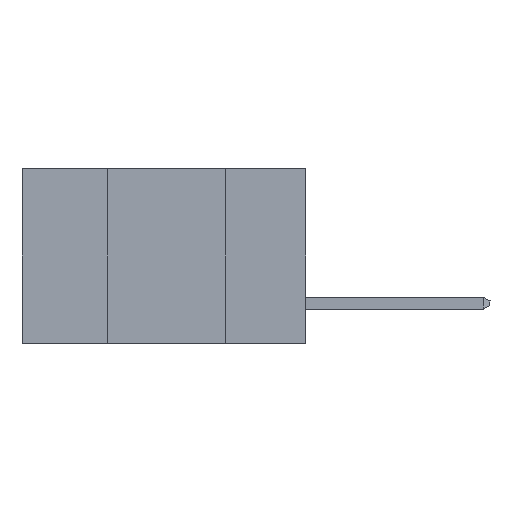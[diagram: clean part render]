
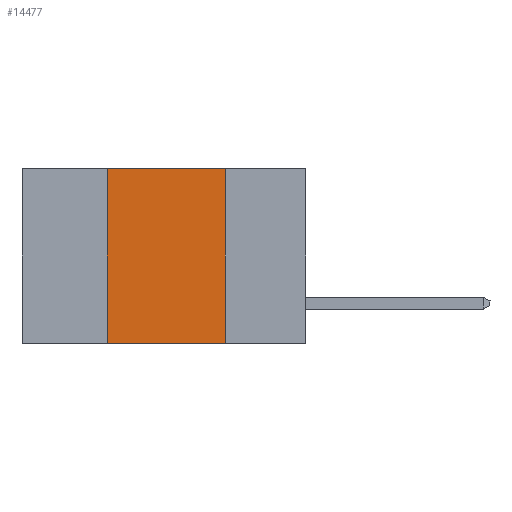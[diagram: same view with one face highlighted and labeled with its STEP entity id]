
A CAD part, left-side view. The second image highlights one B-rep face of the part: STEP entity #14477.
In plain terms, the highlighted planar face has unit normal (-1, 0, 0).
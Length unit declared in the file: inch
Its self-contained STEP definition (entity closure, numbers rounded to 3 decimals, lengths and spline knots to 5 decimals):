
#963 = VECTOR ( 'NONE', #24913, 39.37008 ) ;
#1207 = CARTESIAN_POINT ( 'NONE',  ( 0., 0.6, 0. ) ) ;
#1717 = CARTESIAN_POINT ( 'NONE',  ( 0., 0.17, 0. ) ) ;
#3319 = DIRECTION ( 'NONE',  ( 0., 0., -1. ) ) ;
#4169 = DIRECTION ( 'NONE',  ( 0., 0., -1. ) ) ;
#4294 = VECTOR ( 'NONE', #4169, 39.37008 ) ;
#4435 = CARTESIAN_POINT ( 'NONE',  ( 0., 0.42, 0. ) ) ;
#5025 = EDGE_CURVE ( 'NONE', #22000, #7286, #17313, .T. ) ;
#5263 = DIRECTION ( 'NONE',  ( 0., -1., 0. ) ) ;
#5805 = CARTESIAN_POINT ( 'NONE',  ( 0., 0.17, -0.37 ) ) ;
#7286 = VERTEX_POINT ( 'NONE', #5805 ) ;
#7886 = AXIS2_PLACEMENT_3D ( 'NONE', #11566, #25812, #3319 ) ;
#8017 = CARTESIAN_POINT ( 'NONE',  ( 0., 0.6, -0.37 ) ) ;
#8190 = DIRECTION ( 'NONE',  ( 0., -1., 0. ) ) ;
#8871 = LINE ( 'NONE', #1207, #24539 ) ;
#10489 = EDGE_CURVE ( 'NONE', #13871, #15187, #8871, .T. ) ;
#11566 = CARTESIAN_POINT ( 'NONE',  ( 0., 0.6, 0. ) ) ;
#12592 = LINE ( 'NONE', #1717, #4294 ) ;
#13090 = CARTESIAN_POINT ( 'NONE',  ( 0., 0.42, -0.37 ) ) ;
#13642 = PLANE ( 'NONE',  #7886 ) ;
#13871 = VERTEX_POINT ( 'NONE', #15071 ) ;
#14477 = ADVANCED_FACE ( 'NONE', ( #20947 ), #13642, .F. ) ;
#15071 = CARTESIAN_POINT ( 'NONE',  ( 0., 0.42, 0. ) ) ;
#15187 = VERTEX_POINT ( 'NONE', #24500 ) ;
#15359 = ORIENTED_EDGE ( 'NONE', *, *, #21835, .F. ) ;
#15578 = EDGE_CURVE ( 'NONE', #15187, #7286, #12592, .T. ) ;
#15638 = LINE ( 'NONE', #4435, #963 ) ;
#17313 = LINE ( 'NONE', #8017, #22070 ) ;
#17781 = EDGE_LOOP ( 'NONE', ( #18441, #21659, #15359, #25829 ) ) ;
#18441 = ORIENTED_EDGE ( 'NONE', *, *, #15578, .F. ) ;
#20947 = FACE_OUTER_BOUND ( 'NONE', #17781, .T. ) ;
#21659 = ORIENTED_EDGE ( 'NONE', *, *, #10489, .F. ) ;
#21835 = EDGE_CURVE ( 'NONE', #22000, #13871, #15638, .T. ) ;
#22000 = VERTEX_POINT ( 'NONE', #13090 ) ;
#22070 = VECTOR ( 'NONE', #8190, 39.37008 ) ;
#24500 = CARTESIAN_POINT ( 'NONE',  ( 0., 0.17, 0. ) ) ;
#24539 = VECTOR ( 'NONE', #5263, 39.37008 ) ;
#24913 = DIRECTION ( 'NONE',  ( 0., 0., 1. ) ) ;
#25812 = DIRECTION ( 'NONE',  ( 1., 0., 0. ) ) ;
#25829 = ORIENTED_EDGE ( 'NONE', *, *, #5025, .T. ) ;
